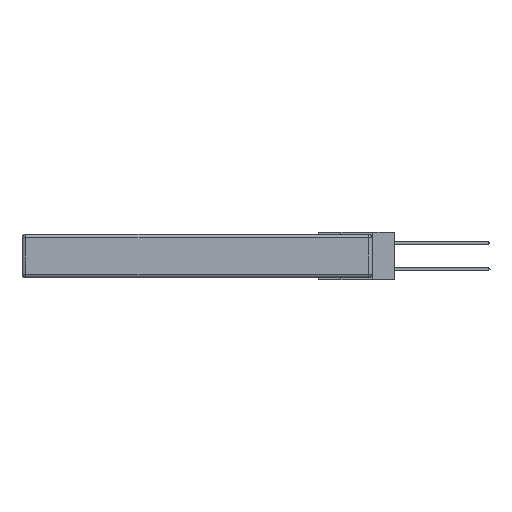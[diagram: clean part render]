
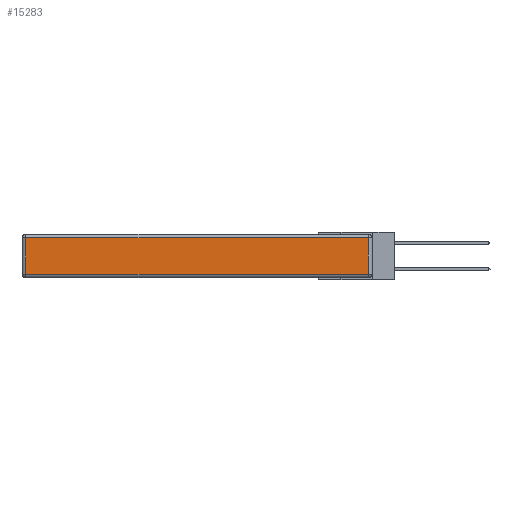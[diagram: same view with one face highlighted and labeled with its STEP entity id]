
A CAD part, left-side view. The second image highlights one B-rep face of the part: STEP entity #15283.
In plain terms, the highlighted planar face has unit normal (-1, 0, 0).
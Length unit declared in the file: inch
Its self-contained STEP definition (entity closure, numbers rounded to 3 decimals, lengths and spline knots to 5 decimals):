
#890 = EDGE_LOOP ( 'NONE', ( #33250, #1217, #8852, #21076 ) ) ;
#976 = DIRECTION ( 'NONE',  ( 0., 1., 0. ) ) ;
#1217 = ORIENTED_EDGE ( 'NONE', *, *, #18573, .T. ) ;
#2144 = VECTOR ( 'NONE', #976, 39.37008 ) ;
#3572 = CARTESIAN_POINT ( 'NONE',  ( 0., 0.03, -0.03 ) ) ;
#4495 = DIRECTION ( 'NONE',  ( 0., -1., 0. ) ) ;
#4567 = CARTESIAN_POINT ( 'NONE',  ( 0., 2.72, -0.313 ) ) ;
#4619 = VERTEX_POINT ( 'NONE', #6648 ) ;
#5422 = CARTESIAN_POINT ( 'NONE',  ( 0., 2.72, -0.03 ) ) ;
#6096 = CARTESIAN_POINT ( 'NONE',  ( 0., 0., -0.343 ) ) ;
#6561 = CARTESIAN_POINT ( 'NONE',  ( 0., 2.75, -0.03 ) ) ;
#6630 = LINE ( 'NONE', #27394, #11457 ) ;
#6648 = CARTESIAN_POINT ( 'NONE',  ( 0., 0.03, -0.313 ) ) ;
#7056 = AXIS2_PLACEMENT_3D ( 'NONE', #6096, #18888, #24077 ) ;
#8320 = VECTOR ( 'NONE', #32878, 39.37008 ) ;
#8852 = ORIENTED_EDGE ( 'NONE', *, *, #12135, .T. ) ;
#8965 = EDGE_CURVE ( 'NONE', #11640, #28718, #23166, .T. ) ;
#9778 = CARTESIAN_POINT ( 'NONE',  ( 0., 2.72, -0.343 ) ) ;
#11457 = VECTOR ( 'NONE', #12180, 39.37008 ) ;
#11640 = VERTEX_POINT ( 'NONE', #5422 ) ;
#12135 = EDGE_CURVE ( 'NONE', #15502, #11640, #26701, .T. ) ;
#12180 = DIRECTION ( 'NONE',  ( 0., 0., 1. ) ) ;
#15283 = ADVANCED_FACE ( 'NONE', ( #23270 ), #16318, .T. ) ;
#15502 = VERTEX_POINT ( 'NONE', #3572 ) ;
#16318 = PLANE ( 'NONE',  #7056 ) ;
#18573 = EDGE_CURVE ( 'NONE', #4619, #15502, #6630, .T. ) ;
#18888 = DIRECTION ( 'NONE',  ( -1., 0., 0. ) ) ;
#21076 = ORIENTED_EDGE ( 'NONE', *, *, #8965, .T. ) ;
#21659 = VECTOR ( 'NONE', #4495, 39.37008 ) ;
#23166 = LINE ( 'NONE', #9778, #8320 ) ;
#23270 = FACE_OUTER_BOUND ( 'NONE', #890, .T. ) ;
#24077 = DIRECTION ( 'NONE',  ( 0., 0., 1. ) ) ;
#24864 = CARTESIAN_POINT ( 'NONE',  ( 0., 0., -0.313 ) ) ;
#26701 = LINE ( 'NONE', #6561, #2144 ) ;
#27394 = CARTESIAN_POINT ( 'NONE',  ( 0., 0.03, -0.343 ) ) ;
#28245 = LINE ( 'NONE', #24864, #21659 ) ;
#28718 = VERTEX_POINT ( 'NONE', #4567 ) ;
#30208 = EDGE_CURVE ( 'NONE', #28718, #4619, #28245, .T. ) ;
#32878 = DIRECTION ( 'NONE',  ( 0., 0., -1. ) ) ;
#33250 = ORIENTED_EDGE ( 'NONE', *, *, #30208, .T. ) ;
